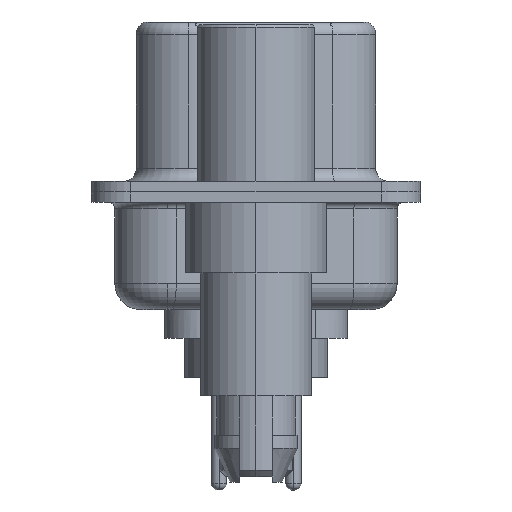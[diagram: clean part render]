
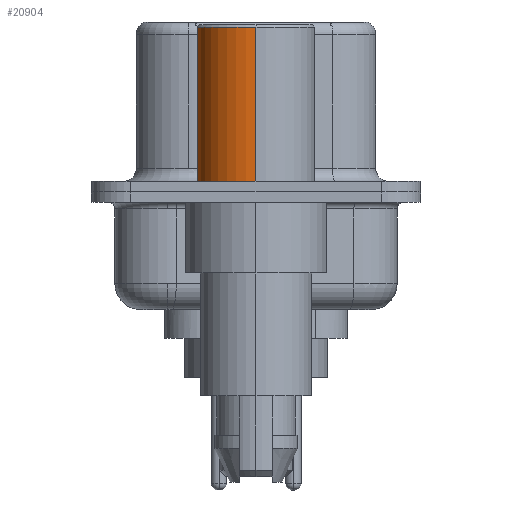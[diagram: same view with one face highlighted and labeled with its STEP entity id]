
A CAD part, left-side view. The second image highlights one B-rep face of the part: STEP entity #20904.
In plain terms, the highlighted cylindrical face has radius 2.25 mm (diameter 4.5 mm), a partial arc.
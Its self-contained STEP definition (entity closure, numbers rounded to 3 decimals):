
#99 = CIRCLE ( 'NONE', #11781, 2.25 ) ;
#900 = EDGE_LOOP ( 'NONE', ( #1474, #14239, #20586, #11925 ) ) ;
#1015 = EDGE_CURVE ( 'NONE', #9363, #19062, #13392, .T. ) ;
#1474 = ORIENTED_EDGE ( 'NONE', *, *, #14836, .T. ) ;
#2537 = AXIS2_PLACEMENT_3D ( 'NONE', #6467, #16593, #14889 ) ;
#2739 = CARTESIAN_POINT ( 'NONE',  ( -2.25, 0., 6.3 ) ) ;
#2932 = CYLINDRICAL_SURFACE ( 'NONE', #2537, 2.25 ) ;
#3103 = DIRECTION ( 'NONE',  ( 0., 0., 1. ) ) ;
#3642 = EDGE_CURVE ( 'NONE', #19062, #21195, #99, .T. ) ;
#4135 = LINE ( 'NONE', #13173, #20989 ) ;
#4421 = VECTOR ( 'NONE', #20512, 1000. ) ;
#5824 = CIRCLE ( 'NONE', #13663, 2.25 ) ;
#6467 = CARTESIAN_POINT ( 'NONE',  ( 0., 0., 0.581 ) ) ;
#7234 = CARTESIAN_POINT ( 'NONE',  ( 0., 0., 0.4 ) ) ;
#7903 = FACE_OUTER_BOUND ( 'NONE', #900, .T. ) ;
#8450 = CARTESIAN_POINT ( 'NONE',  ( 2.25, 0., 0.581 ) ) ;
#8899 = DIRECTION ( 'NONE',  ( 1., 0., 0. ) ) ;
#9363 = VERTEX_POINT ( 'NONE', #18744 ) ;
#9999 = CARTESIAN_POINT ( 'NONE',  ( 0., 0., 6.3 ) ) ;
#10237 = VERTEX_POINT ( 'NONE', #16466 ) ;
#10273 = EDGE_CURVE ( 'NONE', #10237, #21195, #4135, .T. ) ;
#11781 = AXIS2_PLACEMENT_3D ( 'NONE', #9999, #13983, #13898 ) ;
#11925 = ORIENTED_EDGE ( 'NONE', *, *, #1015, .F. ) ;
#13173 = CARTESIAN_POINT ( 'NONE',  ( -2.25, 0., 0.581 ) ) ;
#13392 = LINE ( 'NONE', #8450, #4421 ) ;
#13663 = AXIS2_PLACEMENT_3D ( 'NONE', #7234, #19034, #8899 ) ;
#13898 = DIRECTION ( 'NONE',  ( 1., 0., 0. ) ) ;
#13983 = DIRECTION ( 'NONE',  ( 0., 0., 1. ) ) ;
#14239 = ORIENTED_EDGE ( 'NONE', *, *, #10273, .T. ) ;
#14836 = EDGE_CURVE ( 'NONE', #9363, #10237, #5824, .T. ) ;
#14889 = DIRECTION ( 'NONE',  ( 1., 0., 0. ) ) ;
#16466 = CARTESIAN_POINT ( 'NONE',  ( -2.25, 0., 0.4 ) ) ;
#16593 = DIRECTION ( 'NONE',  ( 0., 0., 1. ) ) ;
#18744 = CARTESIAN_POINT ( 'NONE',  ( 2.25, 0., 0.4 ) ) ;
#19034 = DIRECTION ( 'NONE',  ( 0., 0., 1. ) ) ;
#19062 = VERTEX_POINT ( 'NONE', #19708 ) ;
#19708 = CARTESIAN_POINT ( 'NONE',  ( 2.25, 0., 6.3 ) ) ;
#20512 = DIRECTION ( 'NONE',  ( 0., 0., 1. ) ) ;
#20586 = ORIENTED_EDGE ( 'NONE', *, *, #3642, .F. ) ;
#20904 = ADVANCED_FACE ( 'NONE', ( #7903 ), #2932, .T. ) ;
#20989 = VECTOR ( 'NONE', #3103, 1000. ) ;
#21195 = VERTEX_POINT ( 'NONE', #2739 ) ;
